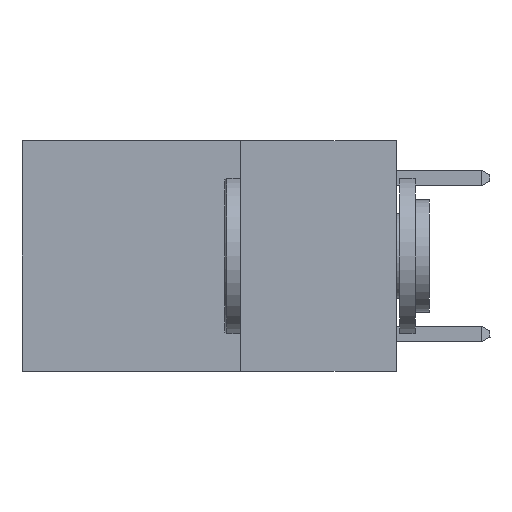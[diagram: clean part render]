
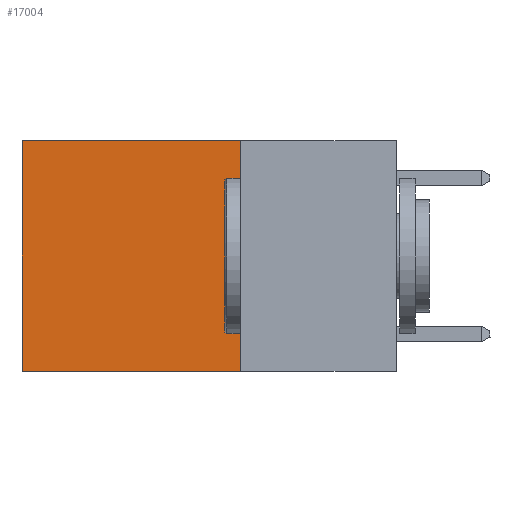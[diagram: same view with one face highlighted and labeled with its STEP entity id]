
A CAD part, left-side view. The second image highlights one B-rep face of the part: STEP entity #17004.
In plain terms, the highlighted planar face has unit normal (-1, 0, 0).
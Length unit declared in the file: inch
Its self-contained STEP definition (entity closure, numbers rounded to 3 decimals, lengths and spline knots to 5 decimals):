
#566 = CARTESIAN_POINT ( 'NONE',  ( 0.2625, 0.25, -0.37 ) ) ;
#769 = ORIENTED_EDGE ( 'NONE', *, *, #18777, .T. ) ;
#814 = ORIENTED_EDGE ( 'NONE', *, *, #18621, .F. ) ;
#867 = VERTEX_POINT ( 'NONE', #18918 ) ;
#1160 = ORIENTED_EDGE ( 'NONE', *, *, #14029, .F. ) ;
#1445 = EDGE_CURVE ( 'NONE', #12852, #16407, #8993, .T. ) ;
#1453 = ORIENTED_EDGE ( 'NONE', *, *, #1445, .T. ) ;
#2857 = CARTESIAN_POINT ( 'NONE',  ( 0.2625, 0.25, 0. ) ) ;
#3922 = DIRECTION ( 'NONE',  ( 1., 0., 0. ) ) ;
#5200 = LINE ( 'NONE', #16577, #5317 ) ;
#5218 = VERTEX_POINT ( 'NONE', #13007 ) ;
#5317 = VECTOR ( 'NONE', #8516, 39.37008 ) ;
#7272 = CARTESIAN_POINT ( 'NONE',  ( 0.2625, 0.25, 0. ) ) ;
#7382 = DIRECTION ( 'NONE',  ( 0., 1., 0. ) ) ;
#7742 = DIRECTION ( 'NONE',  ( 0., 0., -1. ) ) ;
#8516 = DIRECTION ( 'NONE',  ( 0., 0., -1. ) ) ;
#8814 = VECTOR ( 'NONE', #7382, 39.37008 ) ;
#8988 = DIRECTION ( 'NONE',  ( 0., 1., 0. ) ) ;
#8993 = LINE ( 'NONE', #7272, #8814 ) ;
#10912 = AXIS2_PLACEMENT_3D ( 'NONE', #13749, #3922, #15349 ) ;
#12774 = FACE_OUTER_BOUND ( 'NONE', #15116, .T. ) ;
#12852 = VERTEX_POINT ( 'NONE', #2857 ) ;
#13007 = CARTESIAN_POINT ( 'NONE',  ( 0.2625, 0.25, -0.37 ) ) ;
#13749 = CARTESIAN_POINT ( 'NONE',  ( 0.2625, 0.25, 0. ) ) ;
#14029 = EDGE_CURVE ( 'NONE', #12852, #5218, #5200, .T. ) ;
#15116 = EDGE_LOOP ( 'NONE', ( #769, #814, #1160, #1453 ) ) ;
#15349 = DIRECTION ( 'NONE',  ( 0., 0., -1. ) ) ;
#15439 = VECTOR ( 'NONE', #7742, 39.37008 ) ;
#15637 = LINE ( 'NONE', #15859, #15439 ) ;
#15859 = CARTESIAN_POINT ( 'NONE',  ( 0.2625, 0.6, 0. ) ) ;
#16407 = VERTEX_POINT ( 'NONE', #16889 ) ;
#16577 = CARTESIAN_POINT ( 'NONE',  ( 0.2625, 0.25, 0. ) ) ;
#16889 = CARTESIAN_POINT ( 'NONE',  ( 0.2625, 0.6, 0. ) ) ;
#17004 = ADVANCED_FACE ( 'NONE', ( #12774 ), #19832, .F. ) ;
#18621 = EDGE_CURVE ( 'NONE', #5218, #867, #20580, .T. ) ;
#18777 = EDGE_CURVE ( 'NONE', #16407, #867, #15637, .T. ) ;
#18918 = CARTESIAN_POINT ( 'NONE',  ( 0.2625, 0.6, -0.37 ) ) ;
#19832 = PLANE ( 'NONE',  #10912 ) ;
#19919 = VECTOR ( 'NONE', #8988, 39.37008 ) ;
#20580 = LINE ( 'NONE', #566, #19919 ) ;
